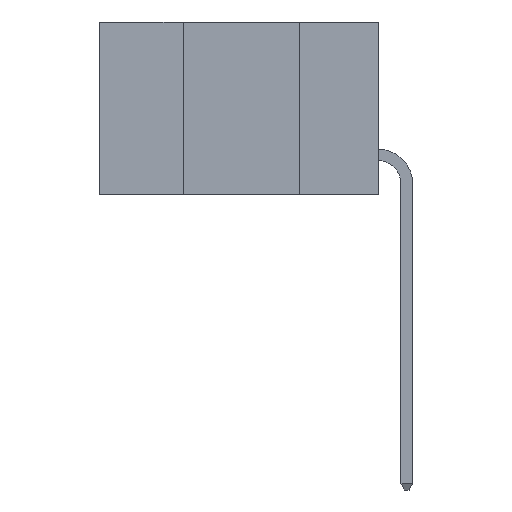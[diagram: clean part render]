
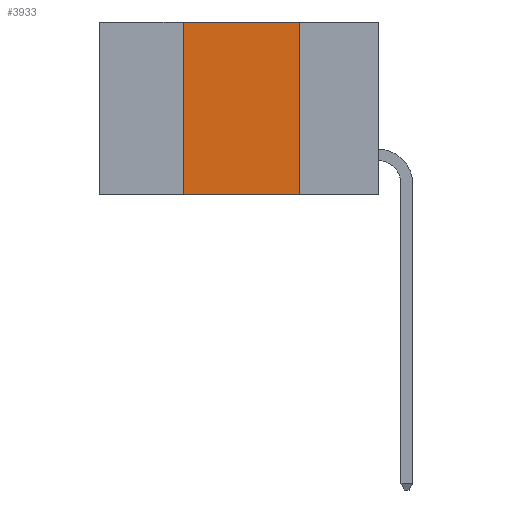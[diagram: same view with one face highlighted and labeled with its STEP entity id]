
A CAD part, left-side view. The second image highlights one B-rep face of the part: STEP entity #3933.
In plain terms, the highlighted planar face has unit normal (-1, 0, 0).
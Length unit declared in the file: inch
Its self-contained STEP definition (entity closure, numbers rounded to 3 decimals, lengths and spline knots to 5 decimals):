
#1186 = VECTOR ( 'NONE', #14587, 39.37008 ) ;
#1300 = CARTESIAN_POINT ( 'NONE',  ( 0., 0.42, -0.37 ) ) ;
#1453 = LINE ( 'NONE', #8001, #11015 ) ;
#2370 = LINE ( 'NONE', #3107, #11369 ) ;
#2828 = CARTESIAN_POINT ( 'NONE',  ( 0., 0.6, -0.37 ) ) ;
#2940 = DIRECTION ( 'NONE',  ( 0., -1., 0. ) ) ;
#3107 = CARTESIAN_POINT ( 'NONE',  ( 0., 0.6, 0. ) ) ;
#3766 = EDGE_CURVE ( 'NONE', #15107, #13221, #2370, .T. ) ;
#3933 = ADVANCED_FACE ( 'NONE', ( #12669 ), #21498, .F. ) ;
#4204 = CARTESIAN_POINT ( 'NONE',  ( 0., 0.42, 0. ) ) ;
#5220 = LINE ( 'NONE', #2828, #1186 ) ;
#5575 = VERTEX_POINT ( 'NONE', #8586 ) ;
#8001 = CARTESIAN_POINT ( 'NONE',  ( 0., 0.17, -0.37 ) ) ;
#8296 = EDGE_LOOP ( 'NONE', ( #11387, #19123, #19601, #16351 ) ) ;
#8586 = CARTESIAN_POINT ( 'NONE',  ( 0., 0.17, -0.37 ) ) ;
#9165 = DIRECTION ( 'NONE',  ( 0., 0., -1. ) ) ;
#9626 = VECTOR ( 'NONE', #16359, 39.37008 ) ;
#10308 = VERTEX_POINT ( 'NONE', #1300 ) ;
#11015 = VECTOR ( 'NONE', #17923, 39.37008 ) ;
#11218 = AXIS2_PLACEMENT_3D ( 'NONE', #21364, #21231, #9165 ) ;
#11369 = VECTOR ( 'NONE', #2940, 39.37008 ) ;
#11387 = ORIENTED_EDGE ( 'NONE', *, *, #12773, .F. ) ;
#12669 = FACE_OUTER_BOUND ( 'NONE', #8296, .T. ) ;
#12773 = EDGE_CURVE ( 'NONE', #13221, #5575, #1453, .T. ) ;
#13122 = CARTESIAN_POINT ( 'NONE',  ( 0., 0.42, -0.37 ) ) ;
#13221 = VERTEX_POINT ( 'NONE', #14053 ) ;
#14053 = CARTESIAN_POINT ( 'NONE',  ( 0., 0.17, 0. ) ) ;
#14587 = DIRECTION ( 'NONE',  ( 0., -1., 0. ) ) ;
#15107 = VERTEX_POINT ( 'NONE', #4204 ) ;
#15244 = EDGE_CURVE ( 'NONE', #10308, #5575, #5220, .T. ) ;
#16351 = ORIENTED_EDGE ( 'NONE', *, *, #15244, .T. ) ;
#16359 = DIRECTION ( 'NONE',  ( 0., 0., 1. ) ) ;
#16482 = EDGE_CURVE ( 'NONE', #10308, #15107, #17901, .T. ) ;
#17901 = LINE ( 'NONE', #13122, #9626 ) ;
#17923 = DIRECTION ( 'NONE',  ( 0., 0., -1. ) ) ;
#19123 = ORIENTED_EDGE ( 'NONE', *, *, #3766, .F. ) ;
#19601 = ORIENTED_EDGE ( 'NONE', *, *, #16482, .F. ) ;
#21231 = DIRECTION ( 'NONE',  ( 1., 0., 0. ) ) ;
#21364 = CARTESIAN_POINT ( 'NONE',  ( 0., 0.6, 0. ) ) ;
#21498 = PLANE ( 'NONE',  #11218 ) ;
